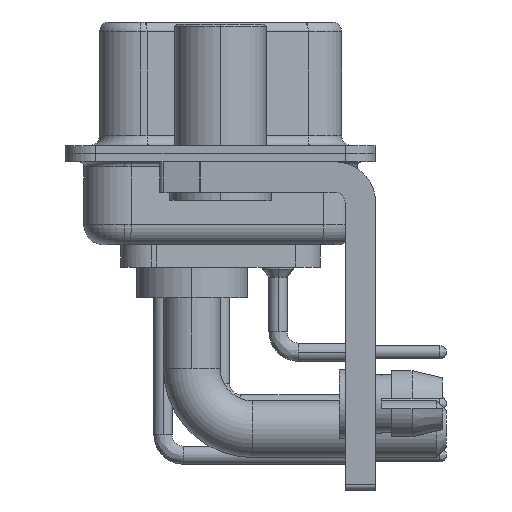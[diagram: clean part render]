
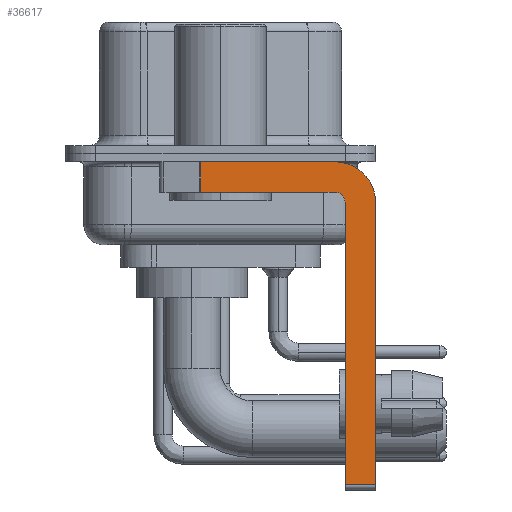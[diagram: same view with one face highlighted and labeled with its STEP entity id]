
A CAD part, left-side view. The second image highlights one B-rep face of the part: STEP entity #36617.
In plain terms, the highlighted planar face has unit normal (-1, 0, 0).
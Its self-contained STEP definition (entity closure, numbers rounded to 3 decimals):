
#847 = LINE ( 'NONE', #20958, #980 ) ;
#980 = VECTOR ( 'NONE', #27426, 1000. ) ;
#1695 = VERTEX_POINT ( 'NONE', #12855 ) ;
#2991 = VECTOR ( 'NONE', #24725, 1000. ) ;
#3408 = VERTEX_POINT ( 'NONE', #24671 ) ;
#4119 = ORIENTED_EDGE ( 'NONE', *, *, #11730, .F. ) ;
#4991 = CARTESIAN_POINT ( 'NONE',  ( -2.9, -5.65, -16.35 ) ) ;
#5416 = DIRECTION ( 'NONE',  ( 1., 0., 0. ) ) ;
#5697 = DIRECTION ( 'NONE',  ( 0., 0., 1. ) ) ;
#6122 = ORIENTED_EDGE ( 'NONE', *, *, #36926, .T. ) ;
#6761 = ORIENTED_EDGE ( 'NONE', *, *, #32009, .F. ) ;
#6995 = VERTEX_POINT ( 'NONE', #24514 ) ;
#7803 = ORIENTED_EDGE ( 'NONE', *, *, #32176, .F. ) ;
#8583 = DIRECTION ( 'NONE',  ( -1., 0., 0. ) ) ;
#9714 = EDGE_CURVE ( 'NONE', #36816, #13684, #31159, .T. ) ;
#10276 = AXIS2_PLACEMENT_3D ( 'NONE', #23674, #8583, #5697 ) ;
#10776 = CARTESIAN_POINT ( 'NONE',  ( -2.9, -5.65, -2.4 ) ) ;
#10891 = VECTOR ( 'NONE', #30133, 1000. ) ;
#11097 = DIRECTION ( 'NONE',  ( 0., -1., 0. ) ) ;
#11730 = EDGE_CURVE ( 'NONE', #6995, #15152, #847, .T. ) ;
#12170 = VECTOR ( 'NONE', #25446, 1000. ) ;
#12855 = CARTESIAN_POINT ( 'NONE',  ( -2.9, 0.978, -0.4 ) ) ;
#13093 = LINE ( 'NONE', #35784, #2991 ) ;
#13150 = LINE ( 'NONE', #21192, #10891 ) ;
#13556 = ORIENTED_EDGE ( 'NONE', *, *, #18090, .F. ) ;
#13631 = VECTOR ( 'NONE', #16167, 1000. ) ;
#13684 = VERTEX_POINT ( 'NONE', #17883 ) ;
#14902 = EDGE_CURVE ( 'NONE', #33509, #3408, #19408, .T. ) ;
#15152 = VERTEX_POINT ( 'NONE', #17047 ) ;
#16167 = DIRECTION ( 'NONE',  ( 0., 0., -1. ) ) ;
#16987 = AXIS2_PLACEMENT_3D ( 'NONE', #10776, #5416, #22446 ) ;
#17047 = CARTESIAN_POINT ( 'NONE',  ( -2.9, 0.978, -1.9 ) ) ;
#17222 = EDGE_CURVE ( 'NONE', #36816, #19923, #13093, .T. ) ;
#17883 = CARTESIAN_POINT ( 'NONE',  ( -2.9, -7.65, -16.35 ) ) ;
#18090 = EDGE_CURVE ( 'NONE', #1695, #33509, #37226, .T. ) ;
#19408 = CIRCLE ( 'NONE', #16987, 2. ) ;
#19923 = VERTEX_POINT ( 'NONE', #32984 ) ;
#20958 = CARTESIAN_POINT ( 'NONE',  ( -2.9, -5.65, -1.9 ) ) ;
#21109 = EDGE_LOOP ( 'NONE', ( #13556, #6122, #4119, #6761, #23821, #30577, #7803, #33348 ) ) ;
#21192 = CARTESIAN_POINT ( 'NONE',  ( -2.9, -7.65, -2.4 ) ) ;
#21906 = LINE ( 'NONE', #33531, #13631 ) ;
#22446 = DIRECTION ( 'NONE',  ( 0., 0., -1. ) ) ;
#23674 = CARTESIAN_POINT ( 'NONE',  ( -2.9, -5.65, -2.4 ) ) ;
#23821 = ORIENTED_EDGE ( 'NONE', *, *, #17222, .F. ) ;
#24514 = CARTESIAN_POINT ( 'NONE',  ( -2.9, -5.65, -1.9 ) ) ;
#24671 = CARTESIAN_POINT ( 'NONE',  ( -2.9, -7.65, -2.4 ) ) ;
#24725 = DIRECTION ( 'NONE',  ( 0., 0., 1. ) ) ;
#25360 = DIRECTION ( 'NONE',  ( 1., 0., 0. ) ) ;
#25446 = DIRECTION ( 'NONE',  ( 0., -1., 0. ) ) ;
#25910 = CARTESIAN_POINT ( 'NONE',  ( -2.9, -5.65, -0.4 ) ) ;
#27426 = DIRECTION ( 'NONE',  ( 0., 1., 0. ) ) ;
#28407 = PLANE ( 'NONE',  #33748 ) ;
#28471 = CARTESIAN_POINT ( 'NONE',  ( -2.9, 3., -0.4 ) ) ;
#29295 = VECTOR ( 'NONE', #11097, 1000. ) ;
#30133 = DIRECTION ( 'NONE',  ( 0., 0., -1. ) ) ;
#30577 = ORIENTED_EDGE ( 'NONE', *, *, #9714, .T. ) ;
#31159 = LINE ( 'NONE', #4991, #12170 ) ;
#31455 = CARTESIAN_POINT ( 'NONE',  ( -2.9, -5.65, -2.4 ) ) ;
#31638 = FACE_OUTER_BOUND ( 'NONE', #21109, .T. ) ;
#32009 = EDGE_CURVE ( 'NONE', #19923, #6995, #33431, .T. ) ;
#32176 = EDGE_CURVE ( 'NONE', #3408, #13684, #13150, .T. ) ;
#32984 = CARTESIAN_POINT ( 'NONE',  ( -2.9, -6.15, -2.4 ) ) ;
#33348 = ORIENTED_EDGE ( 'NONE', *, *, #14902, .F. ) ;
#33431 = CIRCLE ( 'NONE', #10276, 0.5 ) ;
#33509 = VERTEX_POINT ( 'NONE', #25910 ) ;
#33531 = CARTESIAN_POINT ( 'NONE',  ( -2.9, 0.978, -1.9 ) ) ;
#33748 = AXIS2_PLACEMENT_3D ( 'NONE', #31455, #25360, #36976 ) ;
#35784 = CARTESIAN_POINT ( 'NONE',  ( -2.9, -6.15, -16.6 ) ) ;
#36014 = CARTESIAN_POINT ( 'NONE',  ( -2.9, -6.15, -16.35 ) ) ;
#36617 = ADVANCED_FACE ( 'NONE', ( #31638 ), #28407, .F. ) ;
#36816 = VERTEX_POINT ( 'NONE', #36014 ) ;
#36926 = EDGE_CURVE ( 'NONE', #1695, #15152, #21906, .T. ) ;
#36976 = DIRECTION ( 'NONE',  ( 0., 0., -1. ) ) ;
#37226 = LINE ( 'NONE', #28471, #29295 ) ;
